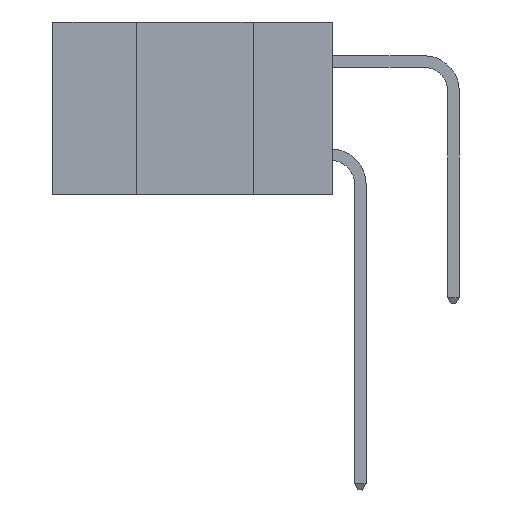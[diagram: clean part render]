
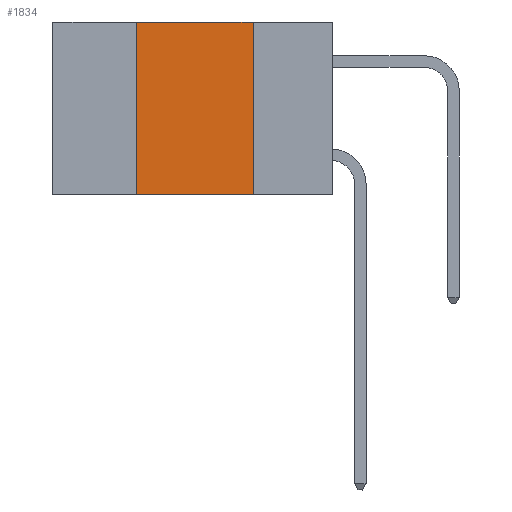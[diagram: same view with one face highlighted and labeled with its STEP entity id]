
A CAD part, left-side view. The second image highlights one B-rep face of the part: STEP entity #1834.
In plain terms, the highlighted planar face has unit normal (-1, 0, 0).
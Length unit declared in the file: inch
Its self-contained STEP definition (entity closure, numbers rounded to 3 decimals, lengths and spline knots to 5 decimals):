
#932 = VECTOR ( 'NONE', #6112, 39.37008 ) ;
#1353 = PLANE ( 'NONE',  #12828 ) ;
#1834 = ADVANCED_FACE ( 'NONE', ( #12622 ), #1353, .F. ) ;
#2141 = ORIENTED_EDGE ( 'NONE', *, *, #3309, .F. ) ;
#2388 = DIRECTION ( 'NONE',  ( 0., 0., 1. ) ) ;
#3309 = EDGE_CURVE ( 'NONE', #10026, #9585, #26122, .T. ) ;
#3371 = LINE ( 'NONE', #20019, #5625 ) ;
#3448 = ORIENTED_EDGE ( 'NONE', *, *, #23336, .F. ) ;
#3849 = LINE ( 'NONE', #14803, #14559 ) ;
#4687 = EDGE_CURVE ( 'NONE', #9585, #8491, #3371, .T. ) ;
#5492 = CARTESIAN_POINT ( 'NONE',  ( 0., 0.6, 0. ) ) ;
#5625 = VECTOR ( 'NONE', #7558, 39.37008 ) ;
#5922 = CARTESIAN_POINT ( 'NONE',  ( 0., 0.17, -0.37 ) ) ;
#6112 = DIRECTION ( 'NONE',  ( 0., -1., 0. ) ) ;
#6132 = CARTESIAN_POINT ( 'NONE',  ( 0., 0.42, 0. ) ) ;
#6294 = ORIENTED_EDGE ( 'NONE', *, *, #8456, .T. ) ;
#7558 = DIRECTION ( 'NONE',  ( 0., 0., -1. ) ) ;
#7559 = DIRECTION ( 'NONE',  ( 1., 0., 0. ) ) ;
#7843 = CARTESIAN_POINT ( 'NONE',  ( 0., 0.6, -0.37 ) ) ;
#8456 = EDGE_CURVE ( 'NONE', #10896, #8491, #22238, .T. ) ;
#8479 = EDGE_LOOP ( 'NONE', ( #11739, #2141, #3448, #6294 ) ) ;
#8491 = VERTEX_POINT ( 'NONE', #5922 ) ;
#9585 = VERTEX_POINT ( 'NONE', #17656 ) ;
#9603 = CARTESIAN_POINT ( 'NONE',  ( 0., 0.6, 0. ) ) ;
#10026 = VERTEX_POINT ( 'NONE', #6132 ) ;
#10896 = VERTEX_POINT ( 'NONE', #16440 ) ;
#11739 = ORIENTED_EDGE ( 'NONE', *, *, #4687, .F. ) ;
#12622 = FACE_OUTER_BOUND ( 'NONE', #8479, .T. ) ;
#12828 = AXIS2_PLACEMENT_3D ( 'NONE', #5492, #7559, #26219 ) ;
#14559 = VECTOR ( 'NONE', #2388, 39.37008 ) ;
#14803 = CARTESIAN_POINT ( 'NONE',  ( 0., 0.42, 0. ) ) ;
#16440 = CARTESIAN_POINT ( 'NONE',  ( 0., 0.42, -0.37 ) ) ;
#17656 = CARTESIAN_POINT ( 'NONE',  ( 0., 0.17, 0. ) ) ;
#18988 = VECTOR ( 'NONE', #26009, 39.37008 ) ;
#20019 = CARTESIAN_POINT ( 'NONE',  ( 0., 0.17, 0. ) ) ;
#22238 = LINE ( 'NONE', #7843, #932 ) ;
#23336 = EDGE_CURVE ( 'NONE', #10896, #10026, #3849, .T. ) ;
#26009 = DIRECTION ( 'NONE',  ( 0., -1., 0. ) ) ;
#26122 = LINE ( 'NONE', #9603, #18988 ) ;
#26219 = DIRECTION ( 'NONE',  ( 0., 0., -1. ) ) ;
